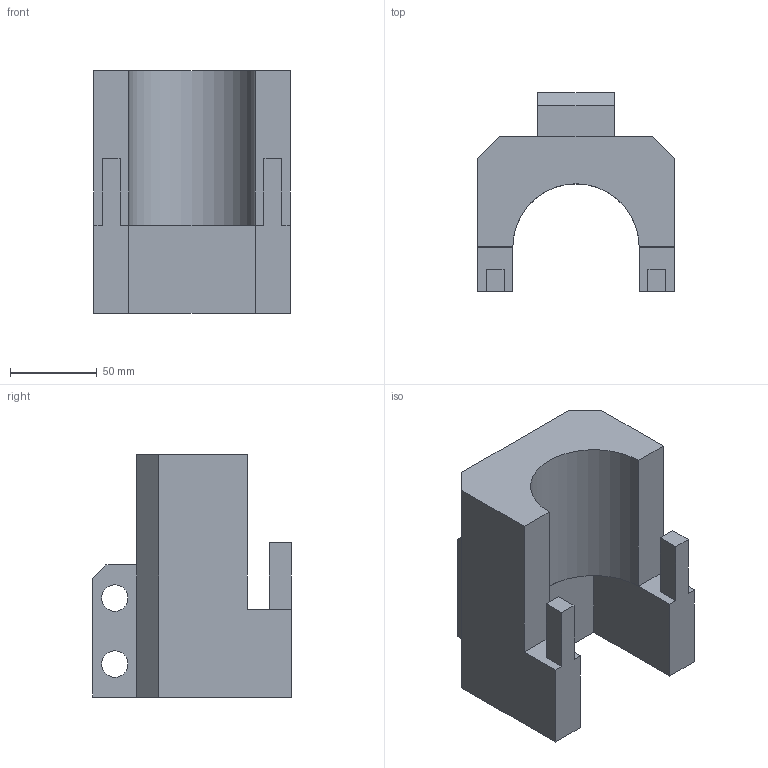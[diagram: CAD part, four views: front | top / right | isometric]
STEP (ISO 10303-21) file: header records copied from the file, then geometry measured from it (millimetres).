
FILE_DESCRIPTION (( 'STEP AP214' ), '1' );
FILE_NAME ('low_retainer.STEP', '2013-09-07T19:05:04', ( '' ), ( '' ), 'SwSTEP 2.0', 'SolidWorks 2013', '' );
FILE_SCHEMA (( 'AUTOMOTIVE_DESIGN' ));
Length unit declared in the file: inch
Products named in the file (1): low_retainer
Bounding box: 113.54 x 114.55 x 139.7 mm (x, y, z)
Volume: 798378.2 mm3; surface area: 84894.1 mm2
Topology: 1 solids, 1 shells, 36 faces, 97 edges, 63 vertices
Faces by surface type: plane 31, cylinder 5
Entity records: 1160 total; most frequent: CARTESIAN_POINT 197, ORIENTED_EDGE 194, DIRECTION 182, EDGE_CURVE 97, VECTOR 86, LINE 86, VERTEX_POINT 63, AXIS2_PLACEMENT_3D 48
